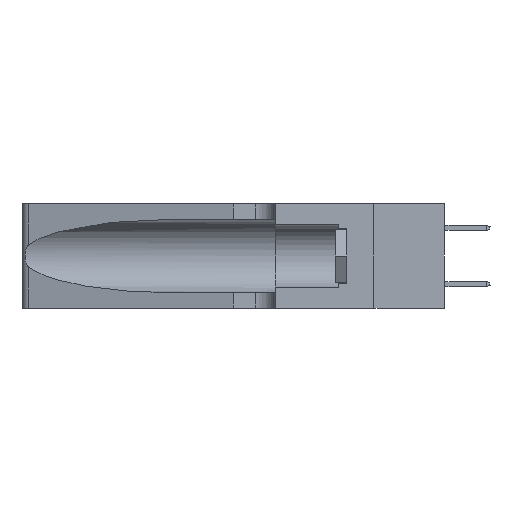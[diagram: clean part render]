
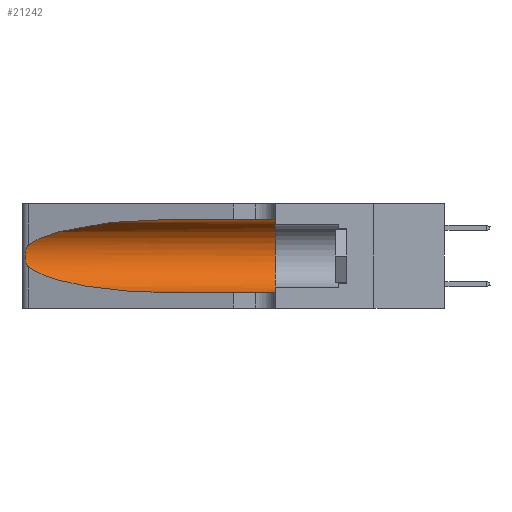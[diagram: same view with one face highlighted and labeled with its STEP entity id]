
A CAD part, left-side view. The second image highlights one B-rep face of the part: STEP entity #21242.
In plain terms, the highlighted cylindrical face has radius 3.308 mm (diameter 6.617 mm), a partial arc.
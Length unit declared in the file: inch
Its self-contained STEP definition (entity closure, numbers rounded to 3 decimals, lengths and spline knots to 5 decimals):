
#342 = AXIS2_PLACEMENT_3D ( 'NONE', #23308, #16636, #25738 ) ;
#1010 = CARTESIAN_POINT ( 'NONE',  ( 0.18966, 0.96281, 0.05475 ) ) ;
#1107 = VECTOR ( 'NONE', #26690, 39.37008 ) ;
#2222 = VERTEX_POINT ( 'NONE', #4888 ) ;
#2711 = CARTESIAN_POINT ( 'NONE',  ( 0.25854, 1.2359, 0.20912 ) ) ;
#3049 = ORIENTED_EDGE ( 'NONE', *, *, #12269, .T. ) ;
#3392 = CARTESIAN_POINT ( 'NONE',  ( 0.2373, 1.15595, 0.28018 ) ) ;
#4888 = CARTESIAN_POINT ( 'NONE',  ( 0.25487, 1.22718, 0.22369 ) ) ;
#4931 = CARTESIAN_POINT ( 'NONE',  ( 0.25639, 1.23186, 0.15144 ) ) ;
#5017 = CARTESIAN_POINT ( 'NONE',  ( 0.25856, 1.23593, 0.16098 ) ) ;
#5207 = CARTESIAN_POINT ( 'NONE',  ( 0.25487, 1.22718, 0.14631 ) ) ;
#5507 = CARTESIAN_POINT ( 'NONE',  ( 0.25487, 1.22718, 0.14631 ) ) ;
#5897 = EDGE_CURVE ( 'NONE', #13975, #22450, #22286, .T. ) ;
#6529 = ORIENTED_EDGE ( 'NONE', *, *, #9041, .F. ) ;
#6530 = CARTESIAN_POINT ( 'NONE',  ( 0.1305, 1.61858, 0.05475 ) ) ;
#7547 = CARTESIAN_POINT ( 'NONE',  ( 0.25487, 1.22718, 0.22369 ) ) ;
#8450 = CARTESIAN_POINT ( 'NONE',  ( 0.1305, 0.35, 0.05475 ) ) ;
#8794 = VERTEX_POINT ( 'NONE', #5507 ) ;
#9041 = EDGE_CURVE ( 'NONE', #21227, #13975, #10504, .T. ) ;
#9514 = CARTESIAN_POINT ( 'NONE',  ( 0.25555, 1.22994, 0.2215 ) ) ;
#9578 = EDGE_CURVE ( 'NONE', #18618, #22450, #27393, .T. ) ;
#10009 = CARTESIAN_POINT ( 'NONE',  ( 0.25487, 1.22718, 0.22369 ) ) ;
#10470 = VECTOR ( 'NONE', #15649, 39.37008 ) ;
#10504 = LINE ( 'NONE', #24294, #1107 ) ;
#10623 =( BOUNDED_CURVE ( )  B_SPLINE_CURVE ( 3, ( #14131, #16337, #1010, #16522 ),
 .UNSPECIFIED., .F., .T. ) 
 B_SPLINE_CURVE_WITH_KNOTS ( ( 4, 4 ),
 ( 3.44316, 4.71239 ),
 .UNSPECIFIED. ) 
 CURVE ( )  GEOMETRIC_REPRESENTATION_ITEM ( )  RATIONAL_B_SPLINE_CURVE ( ( 1., 0.87, 0.87, 1. ) ) 
 REPRESENTATION_ITEM ( '' )  );
#10653 = DIRECTION ( 'NONE',  ( 0., -1., 0. ) ) ;
#10884 = CARTESIAN_POINT ( 'NONE',  ( 0.1305, 0.72297, 0.05475 ) ) ;
#11878 = B_SPLINE_CURVE_WITH_KNOTS ( 'NONE', 3,
 ( #7547, #9514, #15982, #20515, #2711, #13885, #27192, #14068, #16269, #5017, #22939, #4931, #22751, #5207 ),
 .UNSPECIFIED., .F., .F.,
 ( 4, 2, 2, 2, 2, 2, 4 ),
 ( 0., 0.00027, 0.00053, 0.00107, 0.0016, 0.00187, 0.00214 ),
 .UNSPECIFIED. ) ;
#12269 = EDGE_CURVE ( 'NONE', #8794, #18618, #10623, .T. ) ;
#12341 = ORIENTED_EDGE ( 'NONE', *, *, #25559, .T. ) ;
#13306 = CARTESIAN_POINT ( 'NONE',  ( 0.1305, 0.35, 0.31525 ) ) ;
#13885 = CARTESIAN_POINT ( 'NONE',  ( 0.26018, 1.23835, 0.19895 ) ) ;
#13975 = VERTEX_POINT ( 'NONE', #13306 ) ;
#14068 = CARTESIAN_POINT ( 'NONE',  ( 0.26075, 1.23896, 0.178 ) ) ;
#14131 = CARTESIAN_POINT ( 'NONE',  ( 0.25487, 1.22718, 0.14631 ) ) ;
#14555 = CARTESIAN_POINT ( 'NONE',  ( 0.1305, 0.72297, 0.31525 ) ) ;
#15649 = DIRECTION ( 'NONE',  ( 0., -1., 0. ) ) ;
#15758 =( BOUNDED_CURVE ( )  B_SPLINE_CURVE ( 3, ( #14555, #16771, #3392, #10009 ),
 .UNSPECIFIED., .F., .T. ) 
 B_SPLINE_CURVE_WITH_KNOTS ( ( 4, 4 ),
 ( 1.5708, 2.84003 ),
 .UNSPECIFIED. ) 
 CURVE ( )  GEOMETRIC_REPRESENTATION_ITEM ( )  RATIONAL_B_SPLINE_CURVE ( ( 1., 0.87, 0.87, 1. ) ) 
 REPRESENTATION_ITEM ( '' )  );
#15832 = ORIENTED_EDGE ( 'NONE', *, *, #16263, .T. ) ;
#15982 = CARTESIAN_POINT ( 'NONE',  ( 0.25639, 1.23184, 0.21858 ) ) ;
#16263 = EDGE_CURVE ( 'NONE', #2222, #8794, #11878, .T. ) ;
#16269 = CARTESIAN_POINT ( 'NONE',  ( 0.26017, 1.23833, 0.17102 ) ) ;
#16337 = CARTESIAN_POINT ( 'NONE',  ( 0.2373, 1.15595, 0.08982 ) ) ;
#16522 = CARTESIAN_POINT ( 'NONE',  ( 0.1305, 0.72297, 0.05475 ) ) ;
#16636 = DIRECTION ( 'NONE',  ( 0., 1., 0. ) ) ;
#16771 = CARTESIAN_POINT ( 'NONE',  ( 0.18966, 0.96281, 0.31525 ) ) ;
#17195 = CARTESIAN_POINT ( 'NONE',  ( 0.1305, 1.61858, 0.185 ) ) ;
#17284 = ORIENTED_EDGE ( 'NONE', *, *, #5897, .F. ) ;
#18618 = VERTEX_POINT ( 'NONE', #10884 ) ;
#19175 = FACE_OUTER_BOUND ( 'NONE', #19425, .T. ) ;
#19425 = EDGE_LOOP ( 'NONE', ( #12341, #15832, #3049, #20265, #17284, #6529 ) ) ;
#19606 = CARTESIAN_POINT ( 'NONE',  ( 0.1305, 0.72297, 0.31525 ) ) ;
#20265 = ORIENTED_EDGE ( 'NONE', *, *, #9578, .T. ) ;
#20515 = CARTESIAN_POINT ( 'NONE',  ( 0.25787, 1.23484, 0.2124 ) ) ;
#21227 = VERTEX_POINT ( 'NONE', #19606 ) ;
#21242 = ADVANCED_FACE ( 'NONE', ( #19175 ), #22646, .F. ) ;
#22286 = CIRCLE ( 'NONE', #342, 0.13025 ) ;
#22450 = VERTEX_POINT ( 'NONE', #8450 ) ;
#22646 = CYLINDRICAL_SURFACE ( 'NONE', #26506, 0.13025 ) ;
#22751 = CARTESIAN_POINT ( 'NONE',  ( 0.25555, 1.22993, 0.14849 ) ) ;
#22939 = CARTESIAN_POINT ( 'NONE',  ( 0.25789, 1.23486, 0.15765 ) ) ;
#23308 = CARTESIAN_POINT ( 'NONE',  ( 0.1305, 0.35, 0.185 ) ) ;
#24294 = CARTESIAN_POINT ( 'NONE',  ( 0.1305, 1.61858, 0.31525 ) ) ;
#25559 = EDGE_CURVE ( 'NONE', #21227, #2222, #15758, .T. ) ;
#25738 = DIRECTION ( 'NONE',  ( 0., 0., 1. ) ) ;
#26506 = AXIS2_PLACEMENT_3D ( 'NONE', #17195, #10653, #28335 ) ;
#26690 = DIRECTION ( 'NONE',  ( 0., -1., 0. ) ) ;
#27192 = CARTESIAN_POINT ( 'NONE',  ( 0.26075, 1.23896, 0.19203 ) ) ;
#27393 = LINE ( 'NONE', #6530, #10470 ) ;
#28335 = DIRECTION ( 'NONE',  ( 0., 0., -1. ) ) ;
